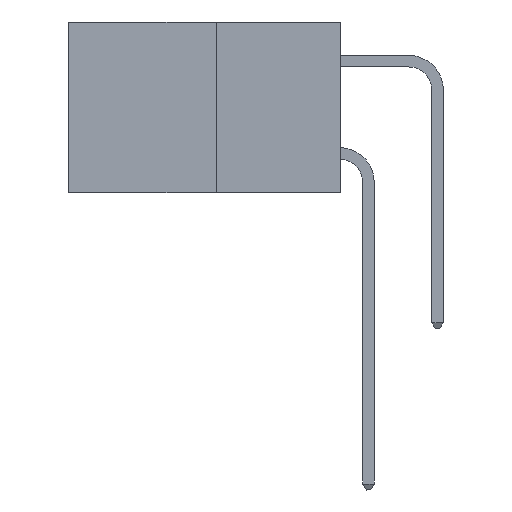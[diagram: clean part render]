
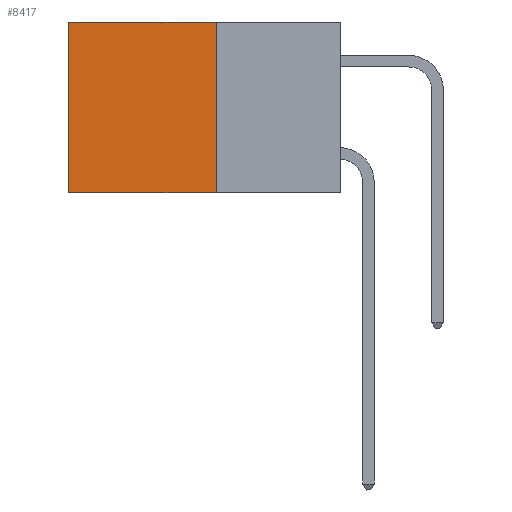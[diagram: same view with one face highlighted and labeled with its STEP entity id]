
A CAD part, left-side view. The second image highlights one B-rep face of the part: STEP entity #8417.
In plain terms, the highlighted planar face has unit normal (-1, 0, 0).
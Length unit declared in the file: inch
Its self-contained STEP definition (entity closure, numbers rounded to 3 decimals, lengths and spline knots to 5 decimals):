
#94 = LINE ( 'NONE', #12733, #4784 ) ;
#163 = FACE_OUTER_BOUND ( 'NONE', #16848, .T. ) ;
#1314 = DIRECTION ( 'NONE',  ( 0., 0., -1. ) ) ;
#1947 = PLANE ( 'NONE',  #26553 ) ;
#1948 = DIRECTION ( 'NONE',  ( 0., 1., 0. ) ) ;
#3111 = ORIENTED_EDGE ( 'NONE', *, *, #28310, .T. ) ;
#4095 = EDGE_CURVE ( 'NONE', #14774, #19677, #21021, .T. ) ;
#4163 = CARTESIAN_POINT ( 'NONE',  ( 0.277, 0.27, -0.37 ) ) ;
#4521 = VERTEX_POINT ( 'NONE', #26041 ) ;
#4784 = VECTOR ( 'NONE', #17354, 39.37008 ) ;
#5398 = VERTEX_POINT ( 'NONE', #28113 ) ;
#6473 = DIRECTION ( 'NONE',  ( 0., 0., -1. ) ) ;
#6576 = DIRECTION ( 'NONE',  ( 1., 0., 0. ) ) ;
#8417 = ADVANCED_FACE ( 'NONE', ( #163 ), #1947, .F. ) ;
#8481 = VECTOR ( 'NONE', #1314, 39.37008 ) ;
#10811 = CARTESIAN_POINT ( 'NONE',  ( 0.277, 0.59, -0.37 ) ) ;
#12431 = VECTOR ( 'NONE', #6473, 39.37008 ) ;
#12506 = EDGE_CURVE ( 'NONE', #4521, #19677, #94, .T. ) ;
#12733 = CARTESIAN_POINT ( 'NONE',  ( 0.277, 0.27, -0.37 ) ) ;
#14774 = VERTEX_POINT ( 'NONE', #22378 ) ;
#16459 = LINE ( 'NONE', #29950, #28154 ) ;
#16848 = EDGE_LOOP ( 'NONE', ( #19710, #18612, #28811, #3111 ) ) ;
#17191 = LINE ( 'NONE', #4163, #12431 ) ;
#17354 = DIRECTION ( 'NONE',  ( 0., 1., 0. ) ) ;
#18612 = ORIENTED_EDGE ( 'NONE', *, *, #12506, .F. ) ;
#19677 = VERTEX_POINT ( 'NONE', #10811 ) ;
#19710 = ORIENTED_EDGE ( 'NONE', *, *, #4095, .T. ) ;
#21021 = LINE ( 'NONE', #28840, #8481 ) ;
#22378 = CARTESIAN_POINT ( 'NONE',  ( 0.277, 0.59, 0. ) ) ;
#23049 = DIRECTION ( 'NONE',  ( 0., 0., -1. ) ) ;
#26041 = CARTESIAN_POINT ( 'NONE',  ( 0.277, 0.27, -0.37 ) ) ;
#26553 = AXIS2_PLACEMENT_3D ( 'NONE', #27661, #6576, #23049 ) ;
#27661 = CARTESIAN_POINT ( 'NONE',  ( 0.277, 0.27, -0.37 ) ) ;
#28113 = CARTESIAN_POINT ( 'NONE',  ( 0.277, 0.27, 0. ) ) ;
#28154 = VECTOR ( 'NONE', #1948, 39.37008 ) ;
#28298 = EDGE_CURVE ( 'NONE', #5398, #4521, #17191, .T. ) ;
#28310 = EDGE_CURVE ( 'NONE', #5398, #14774, #16459, .T. ) ;
#28811 = ORIENTED_EDGE ( 'NONE', *, *, #28298, .F. ) ;
#28840 = CARTESIAN_POINT ( 'NONE',  ( 0.277, 0.59, -0.37 ) ) ;
#29950 = CARTESIAN_POINT ( 'NONE',  ( 0.277, 0.27, 0. ) ) ;
